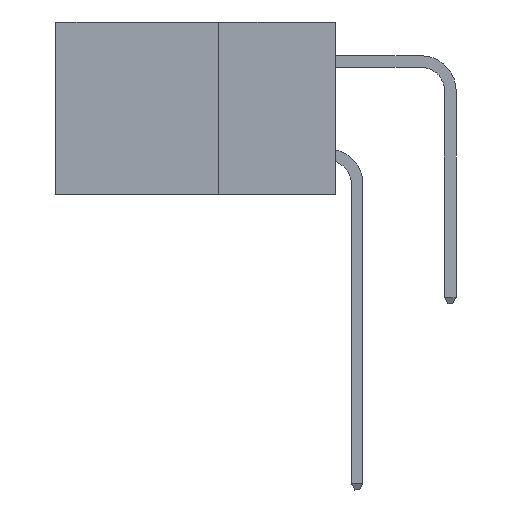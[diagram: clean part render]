
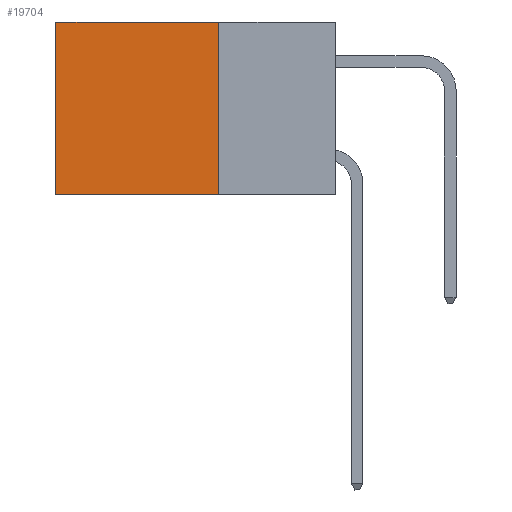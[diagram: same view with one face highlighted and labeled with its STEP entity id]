
A CAD part, left-side view. The second image highlights one B-rep face of the part: STEP entity #19704.
In plain terms, the highlighted planar face has unit normal (-1, 0, 0).
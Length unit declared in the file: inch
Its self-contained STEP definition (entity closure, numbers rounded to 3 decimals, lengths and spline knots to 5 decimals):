
#1805 = ORIENTED_EDGE ( 'NONE', *, *, #21190, .F. ) ;
#2089 = DIRECTION ( 'NONE',  ( 1., 0., 0. ) ) ;
#4065 = AXIS2_PLACEMENT_3D ( 'NONE', #28148, #2089, #7879 ) ;
#4207 = LINE ( 'NONE', #34382, #20203 ) ;
#7224 = DIRECTION ( 'NONE',  ( 0., 0., -1. ) ) ;
#7879 = DIRECTION ( 'NONE',  ( 0., 0., -1. ) ) ;
#8973 = LINE ( 'NONE', #42896, #33121 ) ;
#9636 = VECTOR ( 'NONE', #24082, 39.37008 ) ;
#10095 = CARTESIAN_POINT ( 'NONE',  ( 0.2875, 0.6, 0. ) ) ;
#14168 = CARTESIAN_POINT ( 'NONE',  ( 0.2875, 0.6, 0. ) ) ;
#14686 = EDGE_CURVE ( 'NONE', #19295, #19300, #4207, .T. ) ;
#14850 = VECTOR ( 'NONE', #7224, 39.37008 ) ;
#19295 = VERTEX_POINT ( 'NONE', #27982 ) ;
#19300 = VERTEX_POINT ( 'NONE', #34801 ) ;
#19704 = ADVANCED_FACE ( 'NONE', ( #32263 ), #40940, .F. ) ;
#20203 = VECTOR ( 'NONE', #26919, 39.37008 ) ;
#21190 = EDGE_CURVE ( 'NONE', #19300, #22320, #8973, .T. ) ;
#22320 = VERTEX_POINT ( 'NONE', #41797 ) ;
#23063 = EDGE_CURVE ( 'NONE', #19295, #24394, #27170, .T. ) ;
#24082 = DIRECTION ( 'NONE',  ( 0., 1., 0. ) ) ;
#24394 = VERTEX_POINT ( 'NONE', #14168 ) ;
#25276 = ORIENTED_EDGE ( 'NONE', *, *, #14686, .F. ) ;
#26919 = DIRECTION ( 'NONE',  ( 0., 0., -1. ) ) ;
#27170 = LINE ( 'NONE', #43485, #9636 ) ;
#27408 = EDGE_CURVE ( 'NONE', #24394, #22320, #40928, .T. ) ;
#27982 = CARTESIAN_POINT ( 'NONE',  ( 0.2875, 0.25, 0. ) ) ;
#28148 = CARTESIAN_POINT ( 'NONE',  ( 0.2875, 0.25, 0. ) ) ;
#30076 = ORIENTED_EDGE ( 'NONE', *, *, #27408, .T. ) ;
#30556 = EDGE_LOOP ( 'NONE', ( #30076, #1805, #25276, #31661 ) ) ;
#31661 = ORIENTED_EDGE ( 'NONE', *, *, #23063, .T. ) ;
#32105 = DIRECTION ( 'NONE',  ( 0., 1., 0. ) ) ;
#32263 = FACE_OUTER_BOUND ( 'NONE', #30556, .T. ) ;
#33121 = VECTOR ( 'NONE', #32105, 39.37008 ) ;
#34382 = CARTESIAN_POINT ( 'NONE',  ( 0.2875, 0.25, 0. ) ) ;
#34801 = CARTESIAN_POINT ( 'NONE',  ( 0.2875, 0.25, -0.37 ) ) ;
#40928 = LINE ( 'NONE', #10095, #14850 ) ;
#40940 = PLANE ( 'NONE',  #4065 ) ;
#41797 = CARTESIAN_POINT ( 'NONE',  ( 0.2875, 0.6, -0.37 ) ) ;
#42896 = CARTESIAN_POINT ( 'NONE',  ( 0.2875, 0.25, -0.37 ) ) ;
#43485 = CARTESIAN_POINT ( 'NONE',  ( 0.2875, 0.25, 0. ) ) ;
